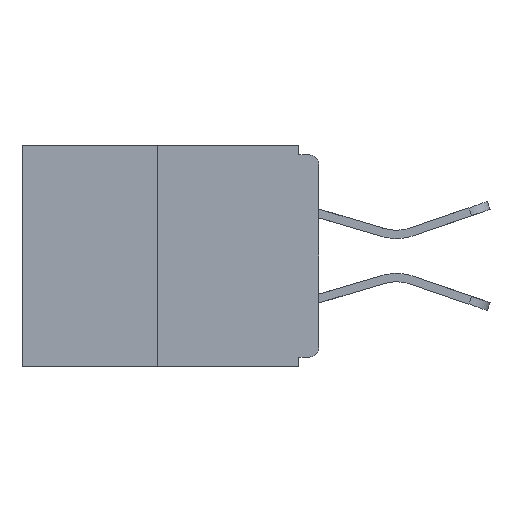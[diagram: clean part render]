
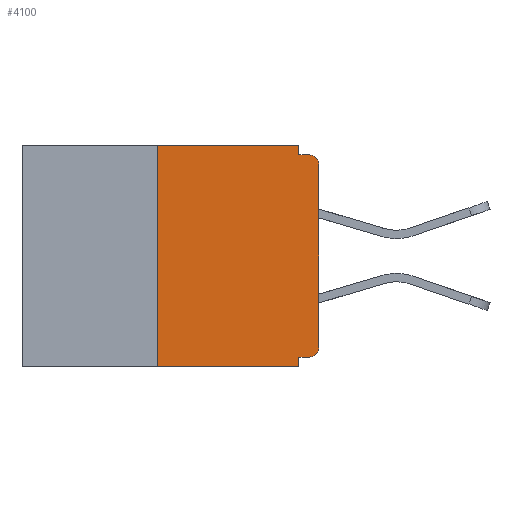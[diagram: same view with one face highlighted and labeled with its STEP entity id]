
A CAD part, left-side view. The second image highlights one B-rep face of the part: STEP entity #4100.
In plain terms, the highlighted planar face has unit normal (-1, 0, 0).
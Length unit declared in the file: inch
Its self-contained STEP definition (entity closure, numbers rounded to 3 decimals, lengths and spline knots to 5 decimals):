
#67 = ORIENTED_EDGE ( 'NONE', *, *, #14943, .T. ) ;
#313 = CARTESIAN_POINT ( 'NONE',  ( 0., 0.031, 0. ) ) ;
#334 = CARTESIAN_POINT ( 'NONE',  ( 0., 0.015, -0.03 ) ) ;
#583 = EDGE_CURVE ( 'NONE', #698, #11698, #17796, .T. ) ;
#698 = VERTEX_POINT ( 'NONE', #2015 ) ;
#911 = ORIENTED_EDGE ( 'NONE', *, *, #13387, .T. ) ;
#1586 = VERTEX_POINT ( 'NONE', #5407 ) ;
#1848 = VECTOR ( 'NONE', #10783, 39.37008 ) ;
#1954 = VECTOR ( 'NONE', #14631, 39.37008 ) ;
#2015 = CARTESIAN_POINT ( 'NONE',  ( 0., 0., -0.313 ) ) ;
#2278 = DIRECTION ( 'NONE',  ( 0., 0., 1. ) ) ;
#2357 = VECTOR ( 'NONE', #15853, 39.37008 ) ;
#2373 = EDGE_CURVE ( 'NONE', #1586, #16000, #8224, .T. ) ;
#2510 = DIRECTION ( 'NONE',  ( -1., 0., 0. ) ) ;
#2777 = CARTESIAN_POINT ( 'NONE',  ( 0., 0.015, -0.313 ) ) ;
#3857 = CARTESIAN_POINT ( 'NONE',  ( 0., 0.46, 0. ) ) ;
#4100 = ADVANCED_FACE ( 'NONE', ( #16990 ), #12899, .F. ) ;
#4423 = VERTEX_POINT ( 'NONE', #11285 ) ;
#4473 = DIRECTION ( 'NONE',  ( 0., 0., -1. ) ) ;
#4476 = DIRECTION ( 'NONE',  ( 0., 0., -1. ) ) ;
#4637 = EDGE_CURVE ( 'NONE', #14786, #4423, #9102, .T. ) ;
#4782 = LINE ( 'NONE', #10543, #13927 ) ;
#4885 = LINE ( 'NONE', #10644, #1954 ) ;
#4943 = VERTEX_POINT ( 'NONE', #18234 ) ;
#5037 = CARTESIAN_POINT ( 'NONE',  ( 0., 0.015, -0.015 ) ) ;
#5127 = AXIS2_PLACEMENT_3D ( 'NONE', #2777, #2510, #14034 ) ;
#5297 = EDGE_CURVE ( 'NONE', #4943, #12472, #4885, .T. ) ;
#5371 = ORIENTED_EDGE ( 'NONE', *, *, #583, .T. ) ;
#5407 = CARTESIAN_POINT ( 'NONE',  ( 0., 0.25, -0.343 ) ) ;
#6028 = ORIENTED_EDGE ( 'NONE', *, *, #5297, .F. ) ;
#6049 = VECTOR ( 'NONE', #13348, 39.37008 ) ;
#6443 = CARTESIAN_POINT ( 'NONE',  ( 0., 0., 0. ) ) ;
#7207 = LINE ( 'NONE', #12974, #12846 ) ;
#7317 = DIRECTION ( 'NONE',  ( -1., 0., 0. ) ) ;
#8035 = CARTESIAN_POINT ( 'NONE',  ( 0., 0.25, 0. ) ) ;
#8207 = LINE ( 'NONE', #10453, #2357 ) ;
#8216 = DIRECTION ( 'NONE',  ( 0., 0., -1. ) ) ;
#8224 = LINE ( 'NONE', #8035, #18181 ) ;
#8225 = LINE ( 'NONE', #16898, #14148 ) ;
#8717 = CARTESIAN_POINT ( 'NONE',  ( 0., 0.031, -0.328 ) ) ;
#9091 = CIRCLE ( 'NONE', #12410, 0.015 ) ;
#9102 = LINE ( 'NONE', #313, #6049 ) ;
#9193 = EDGE_CURVE ( 'NONE', #12472, #18628, #7207, .T. ) ;
#9229 = ORIENTED_EDGE ( 'NONE', *, *, #2373, .F. ) ;
#9347 = ORIENTED_EDGE ( 'NONE', *, *, #11430, .F. ) ;
#9962 = CARTESIAN_POINT ( 'NONE',  ( 0., 0.25, 0. ) ) ;
#10453 = CARTESIAN_POINT ( 'NONE',  ( 0., 0.46, 0. ) ) ;
#10536 = EDGE_CURVE ( 'NONE', #16000, #14786, #8207, .T. ) ;
#10543 = CARTESIAN_POINT ( 'NONE',  ( 0., 0.46, -0.343 ) ) ;
#10630 = EDGE_LOOP ( 'NONE', ( #17977, #9229, #911, #12055, #6028, #12929, #5371, #67, #9347, #17663 ) ) ;
#10644 = CARTESIAN_POINT ( 'NONE',  ( 0., 0., -0.328 ) ) ;
#10783 = DIRECTION ( 'NONE',  ( 0., 0., 1. ) ) ;
#11285 = CARTESIAN_POINT ( 'NONE',  ( 0., 0.031, -0.015 ) ) ;
#11430 = EDGE_CURVE ( 'NONE', #4423, #17979, #8225, .T. ) ;
#11698 = VERTEX_POINT ( 'NONE', #16242 ) ;
#12055 = ORIENTED_EDGE ( 'NONE', *, *, #9193, .F. ) ;
#12410 = AXIS2_PLACEMENT_3D ( 'NONE', #334, #7317, #4476 ) ;
#12412 = EDGE_CURVE ( 'NONE', #4943, #698, #13252, .T. ) ;
#12472 = VERTEX_POINT ( 'NONE', #8717 ) ;
#12833 = CARTESIAN_POINT ( 'NONE',  ( 0., 0.031, 0. ) ) ;
#12846 = VECTOR ( 'NONE', #4473, 39.37008 ) ;
#12899 = PLANE ( 'NONE',  #15388 ) ;
#12929 = ORIENTED_EDGE ( 'NONE', *, *, #12412, .T. ) ;
#12974 = CARTESIAN_POINT ( 'NONE',  ( 0., 0.031, -0.343 ) ) ;
#13252 = CIRCLE ( 'NONE', #5127, 0.015 ) ;
#13348 = DIRECTION ( 'NONE',  ( 0., 0., -1. ) ) ;
#13387 = EDGE_CURVE ( 'NONE', #1586, #18628, #4782, .T. ) ;
#13897 = DIRECTION ( 'NONE',  ( 0., -1., 0. ) ) ;
#13927 = VECTOR ( 'NONE', #16328, 39.37008 ) ;
#14034 = DIRECTION ( 'NONE',  ( 0., 0., -1. ) ) ;
#14148 = VECTOR ( 'NONE', #13897, 39.37008 ) ;
#14631 = DIRECTION ( 'NONE',  ( 0., 1., 0. ) ) ;
#14786 = VERTEX_POINT ( 'NONE', #12833 ) ;
#14943 = EDGE_CURVE ( 'NONE', #11698, #17979, #9091, .T. ) ;
#15388 = AXIS2_PLACEMENT_3D ( 'NONE', #3857, #15584, #8216 ) ;
#15584 = DIRECTION ( 'NONE',  ( 1., 0., 0. ) ) ;
#15853 = DIRECTION ( 'NONE',  ( 0., -1., 0. ) ) ;
#16000 = VERTEX_POINT ( 'NONE', #9962 ) ;
#16242 = CARTESIAN_POINT ( 'NONE',  ( 0., 0., -0.03 ) ) ;
#16328 = DIRECTION ( 'NONE',  ( 0., -1., 0. ) ) ;
#16898 = CARTESIAN_POINT ( 'NONE',  ( 0., 0., -0.015 ) ) ;
#16990 = FACE_OUTER_BOUND ( 'NONE', #10630, .T. ) ;
#17538 = CARTESIAN_POINT ( 'NONE',  ( 0., 0.031, -0.343 ) ) ;
#17663 = ORIENTED_EDGE ( 'NONE', *, *, #4637, .F. ) ;
#17796 = LINE ( 'NONE', #6443, #1848 ) ;
#17977 = ORIENTED_EDGE ( 'NONE', *, *, #10536, .F. ) ;
#17979 = VERTEX_POINT ( 'NONE', #5037 ) ;
#18181 = VECTOR ( 'NONE', #2278, 39.37008 ) ;
#18234 = CARTESIAN_POINT ( 'NONE',  ( 0., 0.015, -0.328 ) ) ;
#18628 = VERTEX_POINT ( 'NONE', #17538 ) ;
